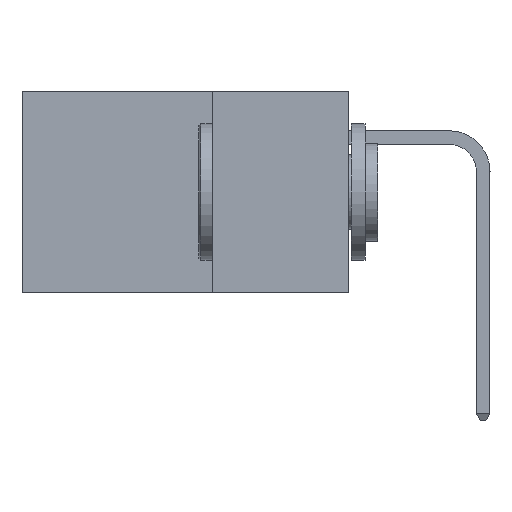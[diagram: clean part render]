
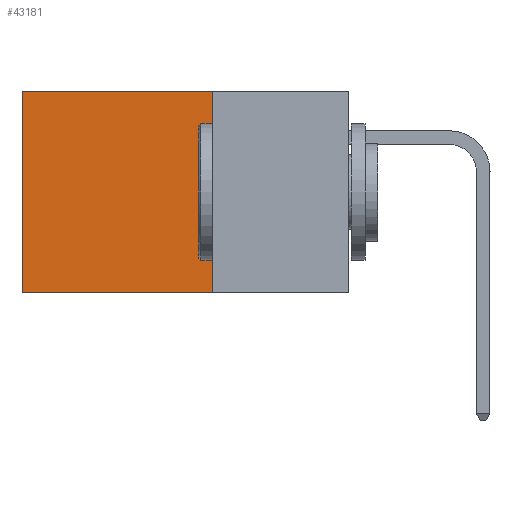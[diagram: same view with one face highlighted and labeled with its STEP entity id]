
A CAD part, left-side view. The second image highlights one B-rep face of the part: STEP entity #43181.
In plain terms, the highlighted planar face has unit normal (-1, 0, 0).
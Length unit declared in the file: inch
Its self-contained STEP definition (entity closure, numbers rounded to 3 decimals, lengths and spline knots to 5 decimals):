
#866 = LINE ( 'NONE', #37859, #27535 ) ;
#2626 = CARTESIAN_POINT ( 'NONE',  ( 0.2875, 0.25, -0.37 ) ) ;
#2734 = CARTESIAN_POINT ( 'NONE',  ( 0.2875, 0.6, 0. ) ) ;
#4572 = CARTESIAN_POINT ( 'NONE',  ( 0.2875, 0.25, 0. ) ) ;
#8769 = CARTESIAN_POINT ( 'NONE',  ( 0.2875, 0.25, -0.37 ) ) ;
#9197 = DIRECTION ( 'NONE',  ( 0., 0., -1. ) ) ;
#9787 = EDGE_LOOP ( 'NONE', ( #26793, #16488, #22739, #27174 ) ) ;
#11808 = LINE ( 'NONE', #8769, #27754 ) ;
#12219 = VERTEX_POINT ( 'NONE', #2734 ) ;
#12722 = DIRECTION ( 'NONE',  ( 0., 1., 0. ) ) ;
#14117 = VECTOR ( 'NONE', #24277, 39.37008 ) ;
#14274 = DIRECTION ( 'NONE',  ( 0., 0., -1. ) ) ;
#16488 = ORIENTED_EDGE ( 'NONE', *, *, #18732, .F. ) ;
#18732 = EDGE_CURVE ( 'NONE', #19805, #33562, #11808, .T. ) ;
#19805 = VERTEX_POINT ( 'NONE', #2626 ) ;
#22074 = EDGE_CURVE ( 'NONE', #28300, #19805, #38576, .T. ) ;
#22739 = ORIENTED_EDGE ( 'NONE', *, *, #22074, .F. ) ;
#24240 = DIRECTION ( 'NONE',  ( 1., 0., 0. ) ) ;
#24277 = DIRECTION ( 'NONE',  ( 0., 0., -1. ) ) ;
#24852 = EDGE_CURVE ( 'NONE', #12219, #33562, #866, .T. ) ;
#25408 = VECTOR ( 'NONE', #12722, 39.37008 ) ;
#26793 = ORIENTED_EDGE ( 'NONE', *, *, #24852, .T. ) ;
#27174 = ORIENTED_EDGE ( 'NONE', *, *, #42924, .T. ) ;
#27535 = VECTOR ( 'NONE', #14274, 39.37008 ) ;
#27754 = VECTOR ( 'NONE', #42762, 39.37008 ) ;
#28300 = VERTEX_POINT ( 'NONE', #33392 ) ;
#29774 = CARTESIAN_POINT ( 'NONE',  ( 0.2875, 0.6, -0.37 ) ) ;
#30484 = CARTESIAN_POINT ( 'NONE',  ( 0.2875, 0.25, 0. ) ) ;
#33392 = CARTESIAN_POINT ( 'NONE',  ( 0.2875, 0.25, 0. ) ) ;
#33562 = VERTEX_POINT ( 'NONE', #29774 ) ;
#33657 = AXIS2_PLACEMENT_3D ( 'NONE', #30484, #24240, #9197 ) ;
#34225 = CARTESIAN_POINT ( 'NONE',  ( 0.2875, 0.25, 0. ) ) ;
#37604 = FACE_OUTER_BOUND ( 'NONE', #9787, .T. ) ;
#37859 = CARTESIAN_POINT ( 'NONE',  ( 0.2875, 0.6, 0. ) ) ;
#38576 = LINE ( 'NONE', #34225, #14117 ) ;
#40443 = PLANE ( 'NONE',  #33657 ) ;
#41873 = LINE ( 'NONE', #4572, #25408 ) ;
#42762 = DIRECTION ( 'NONE',  ( 0., 1., 0. ) ) ;
#42924 = EDGE_CURVE ( 'NONE', #28300, #12219, #41873, .T. ) ;
#43181 = ADVANCED_FACE ( 'NONE', ( #37604 ), #40443, .F. ) ;
